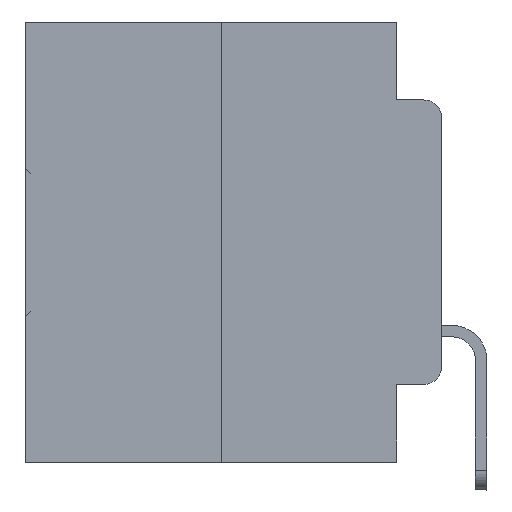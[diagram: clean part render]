
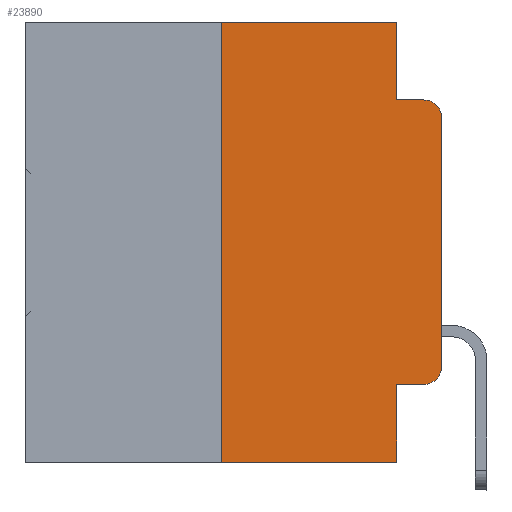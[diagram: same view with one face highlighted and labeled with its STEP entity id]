
A CAD part, left-side view. The second image highlights one B-rep face of the part: STEP entity #23890.
In plain terms, the highlighted planar face has unit normal (-1, 0, 0).
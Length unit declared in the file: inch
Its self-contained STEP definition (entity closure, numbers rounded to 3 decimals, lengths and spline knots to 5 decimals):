
#217 = VERTEX_POINT ( 'NONE', #11231 ) ;
#1933 = LINE ( 'NONE', #31355, #28732 ) ;
#3020 = VECTOR ( 'NONE', #21902, 39.37008 ) ;
#4332 = ORIENTED_EDGE ( 'NONE', *, *, #17790, .F. ) ;
#4447 = AXIS2_PLACEMENT_3D ( 'NONE', #25062, #14763, #22756 ) ;
#5268 = EDGE_CURVE ( 'NONE', #31391, #32754, #6840, .T. ) ;
#5653 = EDGE_CURVE ( 'NONE', #217, #15552, #7187, .T. ) ;
#5668 = EDGE_CURVE ( 'NONE', #31391, #16742, #1933, .T. ) ;
#6840 = LINE ( 'NONE', #24494, #27992 ) ;
#6899 = VECTOR ( 'NONE', #32900, 39.37008 ) ;
#7187 = LINE ( 'NONE', #15360, #33169 ) ;
#9457 = CARTESIAN_POINT ( 'NONE',  ( 0., 0.473, 0. ) ) ;
#9835 = VERTEX_POINT ( 'NONE', #27419 ) ;
#10012 = EDGE_CURVE ( 'NONE', #11236, #32754, #11654, .T. ) ;
#10810 = CIRCLE ( 'NONE', #21217, 0.02 ) ;
#10963 = CIRCLE ( 'NONE', #4447, 0.02 ) ;
#11204 = DIRECTION ( 'NONE',  ( -1., 0., 0. ) ) ;
#11231 = CARTESIAN_POINT ( 'NONE',  ( 0., 0., -0.3915 ) ) ;
#11236 = VERTEX_POINT ( 'NONE', #30573 ) ;
#11550 = EDGE_CURVE ( 'NONE', #11236, #32208, #18882, .T. ) ;
#11654 = LINE ( 'NONE', #12381, #17758 ) ;
#12244 = AXIS2_PLACEMENT_3D ( 'NONE', #30653, #33457, #17973 ) ;
#12381 = CARTESIAN_POINT ( 'NONE',  ( 0., 0.473, -0.5 ) ) ;
#12512 = DIRECTION ( 'NONE',  ( 0., 0., 1. ) ) ;
#12723 = EDGE_LOOP ( 'NONE', ( #18162, #26836, #4332, #18504, #29192, #28847, #26370, #22778, #23999, #26213 ) ) ;
#13414 = DIRECTION ( 'NONE',  ( 0., 0., -1. ) ) ;
#14251 = EDGE_CURVE ( 'NONE', #32208, #32113, #28457, .T. ) ;
#14763 = DIRECTION ( 'NONE',  ( -1., 0., 0. ) ) ;
#15011 = DIRECTION ( 'NONE',  ( 0., -1., 0. ) ) ;
#15360 = CARTESIAN_POINT ( 'NONE',  ( 0., 0., 0. ) ) ;
#15552 = VERTEX_POINT ( 'NONE', #16553 ) ;
#15983 = CARTESIAN_POINT ( 'NONE',  ( 0., 0.02, -0.0885 ) ) ;
#16553 = CARTESIAN_POINT ( 'NONE',  ( 0., 0., -0.1085 ) ) ;
#16662 = VECTOR ( 'NONE', #20718, 39.37008 ) ;
#16742 = VERTEX_POINT ( 'NONE', #28741 ) ;
#17043 = CARTESIAN_POINT ( 'NONE',  ( 0., 0.051, -0.0885 ) ) ;
#17260 = CARTESIAN_POINT ( 'NONE',  ( 0., 0.051, 0. ) ) ;
#17618 = CARTESIAN_POINT ( 'NONE',  ( 0., 0.25, 0. ) ) ;
#17758 = VECTOR ( 'NONE', #15011, 39.37008 ) ;
#17790 = EDGE_CURVE ( 'NONE', #9835, #18642, #26214, .T. ) ;
#17973 = DIRECTION ( 'NONE',  ( 0., 0., -1. ) ) ;
#18162 = ORIENTED_EDGE ( 'NONE', *, *, #5653, .T. ) ;
#18504 = ORIENTED_EDGE ( 'NONE', *, *, #27638, .F. ) ;
#18642 = VERTEX_POINT ( 'NONE', #15983 ) ;
#18882 = LINE ( 'NONE', #17618, #21283 ) ;
#20524 = DIRECTION ( 'NONE',  ( 0., 0., 1. ) ) ;
#20718 = DIRECTION ( 'NONE',  ( 0., 0., -1. ) ) ;
#21010 = CARTESIAN_POINT ( 'NONE',  ( 0., 0.051, -0.4115 ) ) ;
#21217 = AXIS2_PLACEMENT_3D ( 'NONE', #26447, #11204, #13414 ) ;
#21283 = VECTOR ( 'NONE', #12512, 39.37008 ) ;
#21902 = DIRECTION ( 'NONE',  ( 0., -1., 0. ) ) ;
#22756 = DIRECTION ( 'NONE',  ( 0., 0., -1. ) ) ;
#22778 = ORIENTED_EDGE ( 'NONE', *, *, #5268, .F. ) ;
#23890 = ADVANCED_FACE ( 'NONE', ( #28769 ), #28085, .F. ) ;
#23999 = ORIENTED_EDGE ( 'NONE', *, *, #5668, .T. ) ;
#24494 = CARTESIAN_POINT ( 'NONE',  ( 0., 0.051, 0. ) ) ;
#25062 = CARTESIAN_POINT ( 'NONE',  ( 0., 0.02, -0.1085 ) ) ;
#25867 = CARTESIAN_POINT ( 'NONE',  ( 0., 0.051, 0. ) ) ;
#25996 = DIRECTION ( 'NONE',  ( 0., -1., 0. ) ) ;
#26213 = ORIENTED_EDGE ( 'NONE', *, *, #30271, .T. ) ;
#26214 = LINE ( 'NONE', #17043, #3020 ) ;
#26370 = ORIENTED_EDGE ( 'NONE', *, *, #10012, .T. ) ;
#26447 = CARTESIAN_POINT ( 'NONE',  ( 0., 0.02, -0.3915 ) ) ;
#26836 = ORIENTED_EDGE ( 'NONE', *, *, #27447, .T. ) ;
#27419 = CARTESIAN_POINT ( 'NONE',  ( 0., 0.051, -0.0885 ) ) ;
#27447 = EDGE_CURVE ( 'NONE', #15552, #18642, #10963, .T. ) ;
#27638 = EDGE_CURVE ( 'NONE', #32113, #9835, #28816, .T. ) ;
#27992 = VECTOR ( 'NONE', #32385, 39.37008 ) ;
#28085 = PLANE ( 'NONE',  #12244 ) ;
#28457 = LINE ( 'NONE', #9457, #6899 ) ;
#28732 = VECTOR ( 'NONE', #25996, 39.37008 ) ;
#28741 = CARTESIAN_POINT ( 'NONE',  ( 0., 0.02, -0.4115 ) ) ;
#28769 = FACE_OUTER_BOUND ( 'NONE', #12723, .T. ) ;
#28816 = LINE ( 'NONE', #25867, #16662 ) ;
#28847 = ORIENTED_EDGE ( 'NONE', *, *, #11550, .F. ) ;
#29192 = ORIENTED_EDGE ( 'NONE', *, *, #14251, .F. ) ;
#30271 = EDGE_CURVE ( 'NONE', #16742, #217, #10810, .T. ) ;
#30573 = CARTESIAN_POINT ( 'NONE',  ( 0., 0.25, -0.5 ) ) ;
#30653 = CARTESIAN_POINT ( 'NONE',  ( 0., 0.473, 0. ) ) ;
#31355 = CARTESIAN_POINT ( 'NONE',  ( 0., 0.051, -0.4115 ) ) ;
#31391 = VERTEX_POINT ( 'NONE', #21010 ) ;
#32113 = VERTEX_POINT ( 'NONE', #17260 ) ;
#32208 = VERTEX_POINT ( 'NONE', #33482 ) ;
#32385 = DIRECTION ( 'NONE',  ( 0., 0., -1. ) ) ;
#32515 = CARTESIAN_POINT ( 'NONE',  ( 0., 0.051, -0.5 ) ) ;
#32754 = VERTEX_POINT ( 'NONE', #32515 ) ;
#32900 = DIRECTION ( 'NONE',  ( 0., -1., 0. ) ) ;
#33169 = VECTOR ( 'NONE', #20524, 39.37008 ) ;
#33457 = DIRECTION ( 'NONE',  ( 1., 0., 0. ) ) ;
#33482 = CARTESIAN_POINT ( 'NONE',  ( 0., 0.25, 0. ) ) ;
